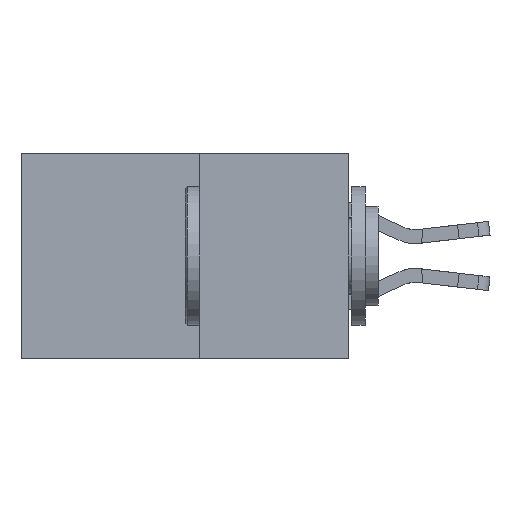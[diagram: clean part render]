
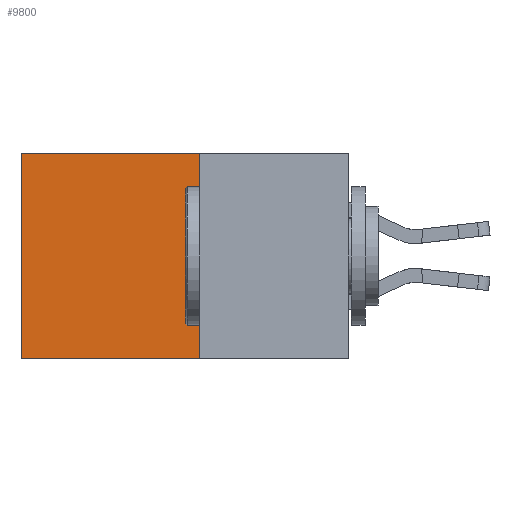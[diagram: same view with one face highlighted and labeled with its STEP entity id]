
A CAD part, left-side view. The second image highlights one B-rep face of the part: STEP entity #9800.
In plain terms, the highlighted planar face has unit normal (-1, 0, 0).
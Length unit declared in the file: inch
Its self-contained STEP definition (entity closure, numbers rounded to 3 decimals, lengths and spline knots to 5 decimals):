
#210 = CARTESIAN_POINT ( 'NONE',  ( 0.277, 0.27, 0. ) ) ;
#656 = ORIENTED_EDGE ( 'NONE', *, *, #1232, .F. ) ;
#1232 = EDGE_CURVE ( 'NONE', #13751, #4466, #11448, .T. ) ;
#1426 = FACE_OUTER_BOUND ( 'NONE', #6525, .T. ) ;
#1476 = DIRECTION ( 'NONE',  ( 0., 1., 0. ) ) ;
#1592 = CARTESIAN_POINT ( 'NONE',  ( 0.277, 0.59, -0.37 ) ) ;
#2417 = CARTESIAN_POINT ( 'NONE',  ( 0.277, 0.27, -0.37 ) ) ;
#3218 = CARTESIAN_POINT ( 'NONE',  ( 0.277, 0.27, -0.37 ) ) ;
#3522 = EDGE_CURVE ( 'NONE', #4324, #13751, #11805, .T. ) ;
#3972 = DIRECTION ( 'NONE',  ( 0., 0., -1. ) ) ;
#4324 = VERTEX_POINT ( 'NONE', #13740 ) ;
#4394 = ORIENTED_EDGE ( 'NONE', *, *, #3522, .F. ) ;
#4466 = VERTEX_POINT ( 'NONE', #12875 ) ;
#4541 = CARTESIAN_POINT ( 'NONE',  ( 0.277, 0.27, -0.37 ) ) ;
#4787 = VECTOR ( 'NONE', #3972, 39.37008 ) ;
#6422 = AXIS2_PLACEMENT_3D ( 'NONE', #3218, #14740, #7972 ) ;
#6520 = VERTEX_POINT ( 'NONE', #10020 ) ;
#6525 = EDGE_LOOP ( 'NONE', ( #9020, #656, #4394, #13570 ) ) ;
#7972 = DIRECTION ( 'NONE',  ( 0., 0., -1. ) ) ;
#8478 = VECTOR ( 'NONE', #10027, 39.37008 ) ;
#8709 = VECTOR ( 'NONE', #1476, 39.37008 ) ;
#9020 = ORIENTED_EDGE ( 'NONE', *, *, #14750, .T. ) ;
#9800 = ADVANCED_FACE ( 'NONE', ( #1426 ), #13590, .F. ) ;
#10020 = CARTESIAN_POINT ( 'NONE',  ( 0.277, 0.59, 0. ) ) ;
#10027 = DIRECTION ( 'NONE',  ( 0., 1., 0. ) ) ;
#11448 = LINE ( 'NONE', #4541, #8478 ) ;
#11805 = LINE ( 'NONE', #13645, #14458 ) ;
#12875 = CARTESIAN_POINT ( 'NONE',  ( 0.277, 0.59, -0.37 ) ) ;
#13567 = DIRECTION ( 'NONE',  ( 0., 0., -1. ) ) ;
#13570 = ORIENTED_EDGE ( 'NONE', *, *, #14658, .T. ) ;
#13590 = PLANE ( 'NONE',  #6422 ) ;
#13645 = CARTESIAN_POINT ( 'NONE',  ( 0.277, 0.27, -0.37 ) ) ;
#13740 = CARTESIAN_POINT ( 'NONE',  ( 0.277, 0.27, 0. ) ) ;
#13751 = VERTEX_POINT ( 'NONE', #2417 ) ;
#13962 = LINE ( 'NONE', #1592, #4787 ) ;
#14458 = VECTOR ( 'NONE', #13567, 39.37008 ) ;
#14658 = EDGE_CURVE ( 'NONE', #4324, #6520, #14672, .T. ) ;
#14672 = LINE ( 'NONE', #210, #8709 ) ;
#14740 = DIRECTION ( 'NONE',  ( 1., 0., 0. ) ) ;
#14750 = EDGE_CURVE ( 'NONE', #6520, #4466, #13962, .T. ) ;
